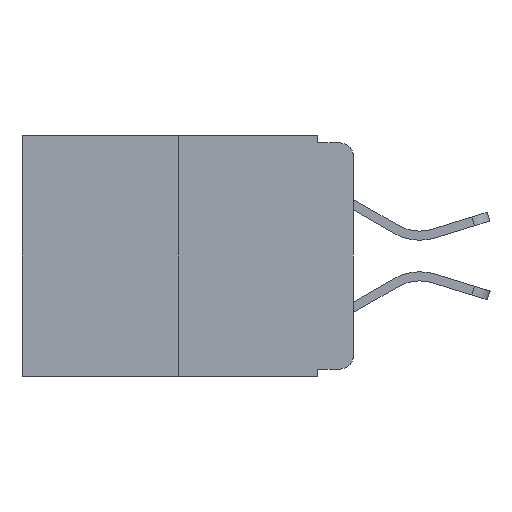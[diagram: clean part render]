
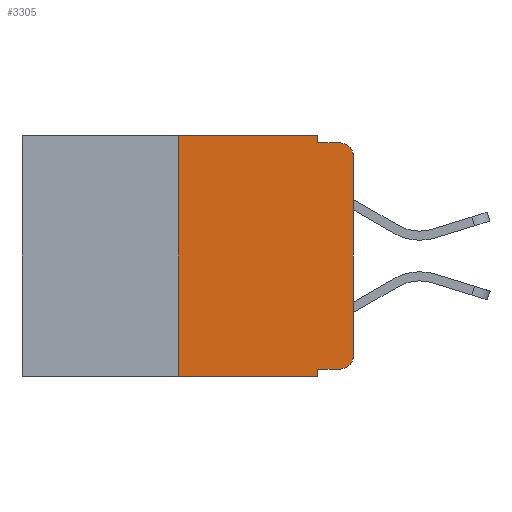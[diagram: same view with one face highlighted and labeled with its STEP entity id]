
A CAD part, left-side view. The second image highlights one B-rep face of the part: STEP entity #3305.
In plain terms, the highlighted planar face has unit normal (-1, 0, 0).
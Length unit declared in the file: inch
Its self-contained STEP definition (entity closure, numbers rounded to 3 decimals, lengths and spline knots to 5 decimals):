
#428 = CARTESIAN_POINT ( 'NONE',  ( 0., 0.051, -0.343 ) ) ;
#505 = ORIENTED_EDGE ( 'NONE', *, *, #5743, .F. ) ;
#582 = DIRECTION ( 'NONE',  ( 0., 0., -1. ) ) ;
#627 = DIRECTION ( 'NONE',  ( 1., 0., 0. ) ) ;
#629 = DIRECTION ( 'NONE',  ( 0., 0., -1. ) ) ;
#691 = DIRECTION ( 'NONE',  ( 0., 0., 1. ) ) ;
#733 = VECTOR ( 'NONE', #4252, 39.37008 ) ;
#751 = DIRECTION ( 'NONE',  ( 0., 0., -1. ) ) ;
#786 = VERTEX_POINT ( 'NONE', #6827 ) ;
#966 = AXIS2_PLACEMENT_3D ( 'NONE', #6360, #6488, #629 ) ;
#1224 = CARTESIAN_POINT ( 'NONE',  ( 0., 0.473, 0. ) ) ;
#1385 = VECTOR ( 'NONE', #8065, 39.37008 ) ;
#1439 = LINE ( 'NONE', #6509, #6617 ) ;
#1459 = CARTESIAN_POINT ( 'NONE',  ( 0., 0.02, -0.01 ) ) ;
#1513 = CARTESIAN_POINT ( 'NONE',  ( 0., 0.473, 0. ) ) ;
#1754 = LINE ( 'NONE', #5233, #8917 ) ;
#2053 = VERTEX_POINT ( 'NONE', #12387 ) ;
#2181 = ORIENTED_EDGE ( 'NONE', *, *, #5895, .F. ) ;
#2276 = VERTEX_POINT ( 'NONE', #8490 ) ;
#2290 = CARTESIAN_POINT ( 'NONE',  ( 0., 0.473, -0.343 ) ) ;
#2464 = CARTESIAN_POINT ( 'NONE',  ( 0., 0.051, -0.333 ) ) ;
#2515 = CARTESIAN_POINT ( 'NONE',  ( 0., 0.051, -0.333 ) ) ;
#2525 = VERTEX_POINT ( 'NONE', #428 ) ;
#2533 = PLANE ( 'NONE',  #3208 ) ;
#2717 = LINE ( 'NONE', #3120, #733 ) ;
#2728 = DIRECTION ( 'NONE',  ( 0., -1., 0. ) ) ;
#3120 = CARTESIAN_POINT ( 'NONE',  ( 0., 0.051, 0. ) ) ;
#3208 = AXIS2_PLACEMENT_3D ( 'NONE', #1513, #627, #582 ) ;
#3287 = DIRECTION ( 'NONE',  ( 0., -1., 0. ) ) ;
#3305 = ADVANCED_FACE ( 'NONE', ( #11108 ), #2533, .F. ) ;
#3482 = DIRECTION ( 'NONE',  ( 0., 0., -1. ) ) ;
#3491 = EDGE_CURVE ( 'NONE', #5716, #12435, #9162, .T. ) ;
#3791 = VECTOR ( 'NONE', #691, 39.37008 ) ;
#3872 = VERTEX_POINT ( 'NONE', #2515 ) ;
#3978 = VECTOR ( 'NONE', #2728, 39.37008 ) ;
#4145 = CARTESIAN_POINT ( 'NONE',  ( 0., 0., -0.03 ) ) ;
#4252 = DIRECTION ( 'NONE',  ( 0., 0., -1. ) ) ;
#4296 = LINE ( 'NONE', #1224, #1385 ) ;
#4372 = ORIENTED_EDGE ( 'NONE', *, *, #6454, .T. ) ;
#4573 = CARTESIAN_POINT ( 'NONE',  ( 0., 0.051, 0. ) ) ;
#4694 = CARTESIAN_POINT ( 'NONE',  ( 0., 0.051, -0.01 ) ) ;
#5233 = CARTESIAN_POINT ( 'NONE',  ( 0., 0.25, 0. ) ) ;
#5716 = VERTEX_POINT ( 'NONE', #10221 ) ;
#5743 = EDGE_CURVE ( 'NONE', #786, #2276, #1754, .T. ) ;
#5895 = EDGE_CURVE ( 'NONE', #3872, #2525, #1439, .T. ) ;
#6342 = ORIENTED_EDGE ( 'NONE', *, *, #3491, .T. ) ;
#6360 = CARTESIAN_POINT ( 'NONE',  ( 0., 0.02, -0.03 ) ) ;
#6454 = EDGE_CURVE ( 'NONE', #3872, #5716, #7385, .T. ) ;
#6479 = CIRCLE ( 'NONE', #966, 0.02 ) ;
#6488 = DIRECTION ( 'NONE',  ( -1., 0., 0. ) ) ;
#6509 = CARTESIAN_POINT ( 'NONE',  ( 0., 0.051, 0. ) ) ;
#6568 = DIRECTION ( 'NONE',  ( -1., 0., 0. ) ) ;
#6617 = VECTOR ( 'NONE', #3482, 39.37008 ) ;
#6827 = CARTESIAN_POINT ( 'NONE',  ( 0., 0.25, -0.343 ) ) ;
#6857 = EDGE_CURVE ( 'NONE', #11194, #2053, #2717, .T. ) ;
#6893 = EDGE_CURVE ( 'NONE', #786, #2525, #7212, .T. ) ;
#7005 = EDGE_CURVE ( 'NONE', #9385, #10900, #6479, .T. ) ;
#7212 = LINE ( 'NONE', #2290, #11318 ) ;
#7385 = LINE ( 'NONE', #2464, #7699 ) ;
#7625 = CARTESIAN_POINT ( 'NONE',  ( 0., 0., -0.313 ) ) ;
#7699 = VECTOR ( 'NONE', #12080, 39.37008 ) ;
#8065 = DIRECTION ( 'NONE',  ( 0., -1., 0. ) ) ;
#8490 = CARTESIAN_POINT ( 'NONE',  ( 0., 0.25, 0. ) ) ;
#8692 = ORIENTED_EDGE ( 'NONE', *, *, #7005, .T. ) ;
#8917 = VECTOR ( 'NONE', #9213, 39.37008 ) ;
#9162 = CIRCLE ( 'NONE', #9285, 0.02 ) ;
#9213 = DIRECTION ( 'NONE',  ( 0., 0., 1. ) ) ;
#9285 = AXIS2_PLACEMENT_3D ( 'NONE', #12389, #6568, #751 ) ;
#9367 = EDGE_CURVE ( 'NONE', #2276, #11194, #4296, .T. ) ;
#9385 = VERTEX_POINT ( 'NONE', #4145 ) ;
#9555 = CARTESIAN_POINT ( 'NONE',  ( 0., 0., 0. ) ) ;
#9629 = EDGE_CURVE ( 'NONE', #2053, #10900, #11288, .T. ) ;
#9811 = ORIENTED_EDGE ( 'NONE', *, *, #9629, .F. ) ;
#10031 = ORIENTED_EDGE ( 'NONE', *, *, #6893, .T. ) ;
#10059 = ORIENTED_EDGE ( 'NONE', *, *, #6857, .F. ) ;
#10221 = CARTESIAN_POINT ( 'NONE',  ( 0., 0.02, -0.333 ) ) ;
#10359 = ORIENTED_EDGE ( 'NONE', *, *, #9367, .F. ) ;
#10900 = VERTEX_POINT ( 'NONE', #1459 ) ;
#11108 = FACE_OUTER_BOUND ( 'NONE', #11825, .T. ) ;
#11188 = EDGE_CURVE ( 'NONE', #12435, #9385, #11858, .T. ) ;
#11194 = VERTEX_POINT ( 'NONE', #4573 ) ;
#11288 = LINE ( 'NONE', #4694, #3978 ) ;
#11318 = VECTOR ( 'NONE', #3287, 39.37008 ) ;
#11338 = ORIENTED_EDGE ( 'NONE', *, *, #11188, .T. ) ;
#11825 = EDGE_LOOP ( 'NONE', ( #11338, #8692, #9811, #10059, #10359, #505, #10031, #2181, #4372, #6342 ) ) ;
#11858 = LINE ( 'NONE', #9555, #3791 ) ;
#12080 = DIRECTION ( 'NONE',  ( 0., -1., 0. ) ) ;
#12387 = CARTESIAN_POINT ( 'NONE',  ( 0., 0.051, -0.01 ) ) ;
#12389 = CARTESIAN_POINT ( 'NONE',  ( 0., 0.02, -0.313 ) ) ;
#12435 = VERTEX_POINT ( 'NONE', #7625 ) ;
